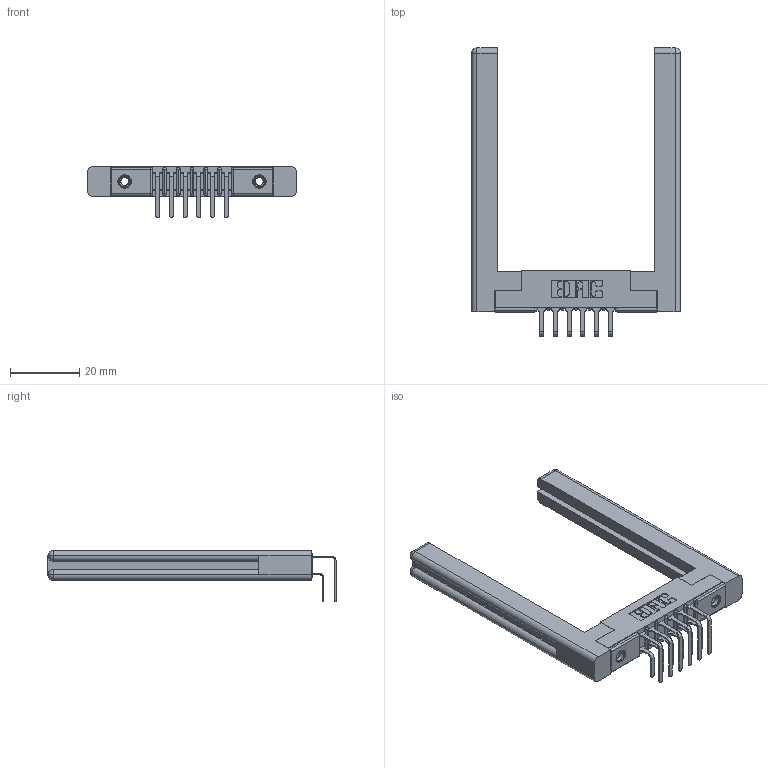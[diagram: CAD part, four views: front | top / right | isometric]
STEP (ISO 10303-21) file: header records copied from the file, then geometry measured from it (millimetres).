
FILE_DESCRIPTION (( 'STEP AP203' ), '1' );
FILE_NAME ('307-012-558-258.STEP', '2019-09-05T18:17:52', ( '' ), ( '' ), 'SwSTEP 2.0', 'SolidWorks 2016', '' );
FILE_SCHEMA (( 'CONFIG_CONTROL_DESIGN' ));
Length unit declared in the file: inch
Products named in the file (6): 307-012-558-258; 307-290-001_558 559 - 1 (Single); 307 Part_.156 Dia Mounting Holes; 345-250-001_345-250-001-102; 307-220-058; 307-290-001_558 - 2 (Single)
Assembly tree (17 placements, depth 2):
  307-012-558-258
    307 Part_.156 Dia Mounting Holes
    307-290-001_558 559 - 1 (Single)  x6
    307-290-001_558 - 2 (Single)  x6
    307-220-058  x2
    345-250-001_345-250-001-102  x2
Bounding box: 60.4 x 83.27 x 14.81 mm (x, y, z)
Volume: 11692.5 mm3; surface area: 11629.9 mm2
Topology: 17 solids, 17 shells, 867 faces, 2381 edges, 1538 vertices
Faces by surface type: plane 550, cylinder 279, sphere 14, torus 12, cone 12
Entity records: 13854 total; most frequent: CARTESIAN_POINT 2299, DIRECTION 2224, ORIENTED_EDGE 2216, EDGE_CURVE 1108, LINE 830, VECTOR 830, VERTEX_POINT 718, AXIS2_PLACEMENT_3D 697
